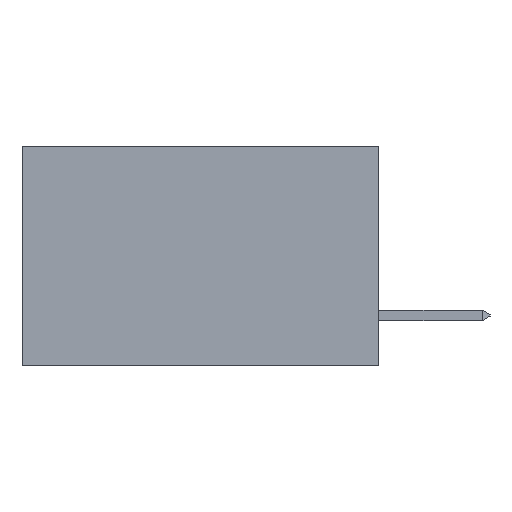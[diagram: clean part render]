
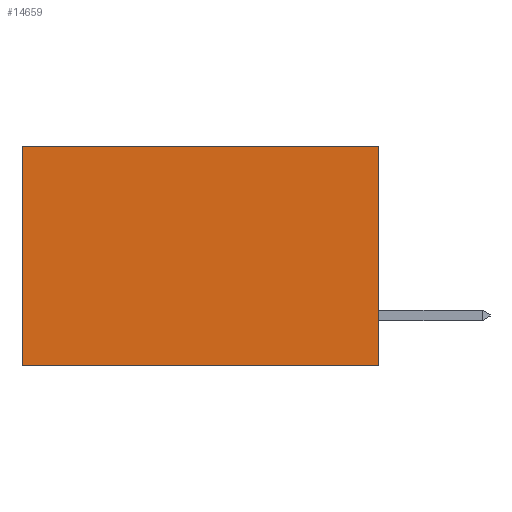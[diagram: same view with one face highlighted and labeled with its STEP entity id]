
A CAD part, left-side view. The second image highlights one B-rep face of the part: STEP entity #14659.
In plain terms, the highlighted planar face has unit normal (-1, 0, 0).
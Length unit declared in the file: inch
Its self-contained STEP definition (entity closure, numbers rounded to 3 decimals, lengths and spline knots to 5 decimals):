
#313 = VECTOR ( 'NONE', #1781, 39.37008 ) ;
#1445 = EDGE_CURVE ( 'NONE', #3044, #4594, #16878, .T. ) ;
#1542 = ORIENTED_EDGE ( 'NONE', *, *, #1445, .T. ) ;
#1781 = DIRECTION ( 'NONE',  ( 0., 1., 0. ) ) ;
#1844 = VECTOR ( 'NONE', #18687, 39.37008 ) ;
#2173 = PLANE ( 'NONE',  #8015 ) ;
#3044 = VERTEX_POINT ( 'NONE', #27382 ) ;
#4590 = CARTESIAN_POINT ( 'NONE',  ( 0.298, 0., 0. ) ) ;
#4594 = VERTEX_POINT ( 'NONE', #28026 ) ;
#5886 = FACE_OUTER_BOUND ( 'NONE', #8582, .T. ) ;
#6618 = CARTESIAN_POINT ( 'NONE',  ( 0.298, 0., 0. ) ) ;
#6660 = VERTEX_POINT ( 'NONE', #16569 ) ;
#7862 = EDGE_CURVE ( 'NONE', #4594, #6660, #14626, .T. ) ;
#8015 = AXIS2_PLACEMENT_3D ( 'NONE', #4590, #26237, #11793 ) ;
#8582 = EDGE_LOOP ( 'NONE', ( #30674, #9642, #27760, #1542 ) ) ;
#9642 = ORIENTED_EDGE ( 'NONE', *, *, #14215, .F. ) ;
#10262 = DIRECTION ( 'NONE',  ( 0., 0., -1. ) ) ;
#11793 = DIRECTION ( 'NONE',  ( 0., 0., -1. ) ) ;
#14215 = EDGE_CURVE ( 'NONE', #26751, #6660, #26635, .T. ) ;
#14626 = LINE ( 'NONE', #28446, #1844 ) ;
#14659 = ADVANCED_FACE ( 'NONE', ( #5886 ), #2173, .F. ) ;
#15473 = DIRECTION ( 'NONE',  ( 0., 1., 0. ) ) ;
#15593 = CARTESIAN_POINT ( 'NONE',  ( 0.298, 0., -0.37 ) ) ;
#16145 = LINE ( 'NONE', #17585, #27426 ) ;
#16569 = CARTESIAN_POINT ( 'NONE',  ( 0.298, 0.6, -0.37 ) ) ;
#16878 = LINE ( 'NONE', #6618, #29580 ) ;
#17585 = CARTESIAN_POINT ( 'NONE',  ( 0.298, 0., 0. ) ) ;
#18687 = DIRECTION ( 'NONE',  ( 0., 0., -1. ) ) ;
#26237 = DIRECTION ( 'NONE',  ( 1., 0., 0. ) ) ;
#26635 = LINE ( 'NONE', #28135, #313 ) ;
#26751 = VERTEX_POINT ( 'NONE', #15593 ) ;
#27382 = CARTESIAN_POINT ( 'NONE',  ( 0.298, 0., 0. ) ) ;
#27426 = VECTOR ( 'NONE', #10262, 39.37008 ) ;
#27760 = ORIENTED_EDGE ( 'NONE', *, *, #29220, .F. ) ;
#28026 = CARTESIAN_POINT ( 'NONE',  ( 0.298, 0.6, 0. ) ) ;
#28135 = CARTESIAN_POINT ( 'NONE',  ( 0.298, 0., -0.37 ) ) ;
#28446 = CARTESIAN_POINT ( 'NONE',  ( 0.298, 0.6, 0. ) ) ;
#29220 = EDGE_CURVE ( 'NONE', #3044, #26751, #16145, .T. ) ;
#29580 = VECTOR ( 'NONE', #15473, 39.37008 ) ;
#30674 = ORIENTED_EDGE ( 'NONE', *, *, #7862, .T. ) ;
